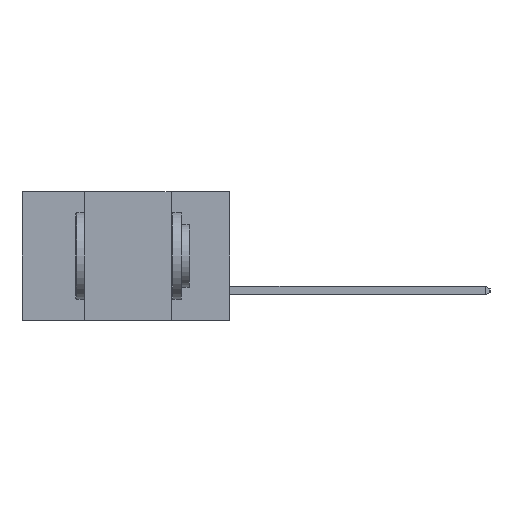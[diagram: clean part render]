
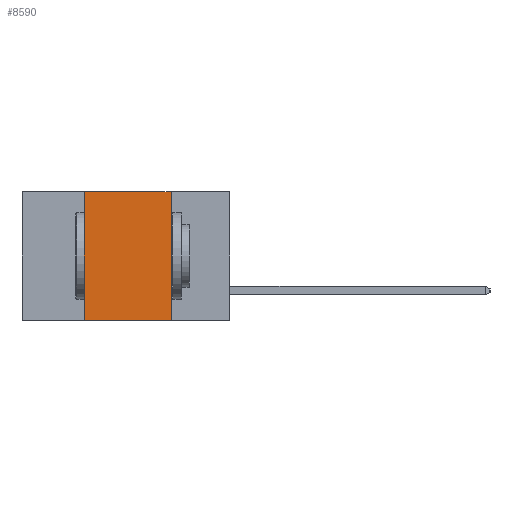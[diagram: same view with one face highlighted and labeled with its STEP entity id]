
A CAD part, left-side view. The second image highlights one B-rep face of the part: STEP entity #8590.
In plain terms, the highlighted planar face has unit normal (-1, 0, 0).
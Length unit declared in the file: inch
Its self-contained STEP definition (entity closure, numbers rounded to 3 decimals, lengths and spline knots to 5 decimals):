
#94 = ORIENTED_EDGE ( 'NONE', *, *, #6234, .F. ) ;
#125 = ORIENTED_EDGE ( 'NONE', *, *, #8608, .T. ) ;
#606 = LINE ( 'NONE', #9626, #8489 ) ;
#637 = LINE ( 'NONE', #9319, #5074 ) ;
#1202 = ORIENTED_EDGE ( 'NONE', *, *, #8022, .F. ) ;
#1396 = PLANE ( 'NONE',  #6916 ) ;
#2328 = VECTOR ( 'NONE', #6642, 39.37008 ) ;
#2964 = VERTEX_POINT ( 'NONE', #3722 ) ;
#3071 = DIRECTION ( 'NONE',  ( 0., 0., -1. ) ) ;
#3159 = VERTEX_POINT ( 'NONE', #9287 ) ;
#3176 = ORIENTED_EDGE ( 'NONE', *, *, #3648, .F. ) ;
#3648 = EDGE_CURVE ( 'NONE', #7590, #2964, #9471, .T. ) ;
#3722 = CARTESIAN_POINT ( 'NONE',  ( 0., 0.17, -0.37 ) ) ;
#4338 = DIRECTION ( 'NONE',  ( 0., -1., 0. ) ) ;
#4532 = LINE ( 'NONE', #5234, #2328 ) ;
#5074 = VECTOR ( 'NONE', #4338, 39.37008 ) ;
#5234 = CARTESIAN_POINT ( 'NONE',  ( 0., 0.42, -0.37 ) ) ;
#6217 = DIRECTION ( 'NONE',  ( 0., -1., 0. ) ) ;
#6234 = EDGE_CURVE ( 'NONE', #3159, #7590, #637, .T. ) ;
#6420 = EDGE_LOOP ( 'NONE', ( #3176, #94, #1202, #125 ) ) ;
#6440 = CARTESIAN_POINT ( 'NONE',  ( 0., 0.42, -0.37 ) ) ;
#6642 = DIRECTION ( 'NONE',  ( 0., 0., 1. ) ) ;
#6767 = CARTESIAN_POINT ( 'NONE',  ( 0., 0.17, 0. ) ) ;
#6852 = CARTESIAN_POINT ( 'NONE',  ( 0., 0.6, 0. ) ) ;
#6916 = AXIS2_PLACEMENT_3D ( 'NONE', #6852, #7538, #3071 ) ;
#7277 = DIRECTION ( 'NONE',  ( 0., 0., -1. ) ) ;
#7351 = CARTESIAN_POINT ( 'NONE',  ( 0., 0.17, -0.37 ) ) ;
#7538 = DIRECTION ( 'NONE',  ( 1., 0., 0. ) ) ;
#7590 = VERTEX_POINT ( 'NONE', #6767 ) ;
#7603 = VECTOR ( 'NONE', #7277, 39.37008 ) ;
#8022 = EDGE_CURVE ( 'NONE', #9483, #3159, #4532, .T. ) ;
#8489 = VECTOR ( 'NONE', #6217, 39.37008 ) ;
#8590 = ADVANCED_FACE ( 'NONE', ( #8726 ), #1396, .F. ) ;
#8608 = EDGE_CURVE ( 'NONE', #9483, #2964, #606, .T. ) ;
#8726 = FACE_OUTER_BOUND ( 'NONE', #6420, .T. ) ;
#9287 = CARTESIAN_POINT ( 'NONE',  ( 0., 0.42, 0. ) ) ;
#9319 = CARTESIAN_POINT ( 'NONE',  ( 0., 0.6, 0. ) ) ;
#9471 = LINE ( 'NONE', #7351, #7603 ) ;
#9483 = VERTEX_POINT ( 'NONE', #6440 ) ;
#9626 = CARTESIAN_POINT ( 'NONE',  ( 0., 0.6, -0.37 ) ) ;
